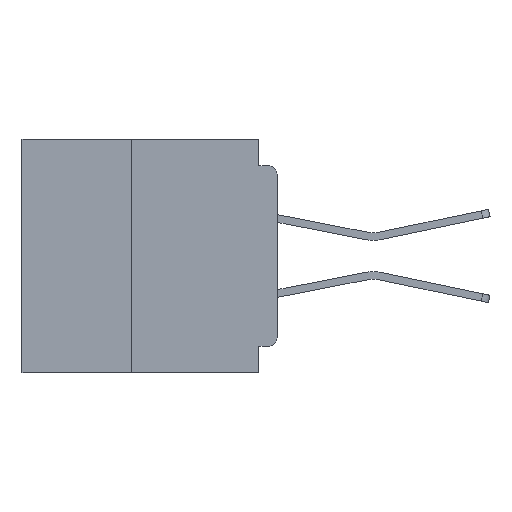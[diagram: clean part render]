
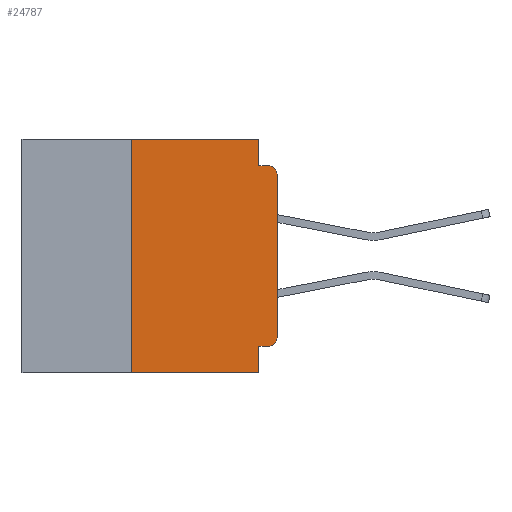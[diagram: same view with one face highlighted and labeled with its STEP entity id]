
A CAD part, left-side view. The second image highlights one B-rep face of the part: STEP entity #24787.
In plain terms, the highlighted planar face has unit normal (-1, 0, 0).
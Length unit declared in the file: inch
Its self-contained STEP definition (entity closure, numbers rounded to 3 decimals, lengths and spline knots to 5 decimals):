
#1979 = VECTOR ( 'NONE', #18012, 39.37008 ) ;
#2396 = EDGE_CURVE ( 'NONE', #15850, #34930, #3824, .T. ) ;
#2592 = VERTEX_POINT ( 'NONE', #10061 ) ;
#2812 = VECTOR ( 'NONE', #30280, 39.37008 ) ;
#2983 = DIRECTION ( 'NONE',  ( 0., -1., 0. ) ) ;
#3063 = ORIENTED_EDGE ( 'NONE', *, *, #26217, .F. ) ;
#3742 = DIRECTION ( 'NONE',  ( 0., -1., 0. ) ) ;
#3824 = LINE ( 'NONE', #6038, #18652 ) ;
#4009 = ORIENTED_EDGE ( 'NONE', *, *, #22475, .F. ) ;
#4136 = DIRECTION ( 'NONE',  ( 0., 0., 1. ) ) ;
#5401 = EDGE_CURVE ( 'NONE', #19291, #34097, #37552, .T. ) ;
#5407 = LINE ( 'NONE', #26726, #20202 ) ;
#5460 = VECTOR ( 'NONE', #17049, 39.37008 ) ;
#5598 = FACE_OUTER_BOUND ( 'NONE', #36679, .T. ) ;
#5671 = CIRCLE ( 'NONE', #7348, 0.015 ) ;
#5683 = VERTEX_POINT ( 'NONE', #23159 ) ;
#5840 = EDGE_CURVE ( 'NONE', #33795, #24374, #13364, .T. ) ;
#5862 = ORIENTED_EDGE ( 'NONE', *, *, #24392, .F. ) ;
#6038 = CARTESIAN_POINT ( 'NONE',  ( 0., 0., -0.045 ) ) ;
#6291 = AXIS2_PLACEMENT_3D ( 'NONE', #11101, #31573, #14049 ) ;
#7348 = AXIS2_PLACEMENT_3D ( 'NONE', #16916, #37301, #19865 ) ;
#8379 = EDGE_CURVE ( 'NONE', #2592, #34930, #5671, .T. ) ;
#8705 = ORIENTED_EDGE ( 'NONE', *, *, #24047, .T. ) ;
#8788 = VECTOR ( 'NONE', #3742, 39.37008 ) ;
#8977 = CIRCLE ( 'NONE', #6291, 0.015 ) ;
#10061 = CARTESIAN_POINT ( 'NONE',  ( 0., 0., -0.06 ) ) ;
#11101 = CARTESIAN_POINT ( 'NONE',  ( 0., 0.015, -0.34 ) ) ;
#11539 = DIRECTION ( 'NONE',  ( 0., 0., -1. ) ) ;
#13364 = LINE ( 'NONE', #17894, #5460 ) ;
#13857 = EDGE_CURVE ( 'NONE', #27856, #2592, #37462, .T. ) ;
#14049 = DIRECTION ( 'NONE',  ( 0., 0., -1. ) ) ;
#15850 = VERTEX_POINT ( 'NONE', #20025 ) ;
#16067 = ORIENTED_EDGE ( 'NONE', *, *, #28334, .F. ) ;
#16609 = LINE ( 'NONE', #24405, #8788 ) ;
#16916 = CARTESIAN_POINT ( 'NONE',  ( 0., 0.015, -0.06 ) ) ;
#17049 = DIRECTION ( 'NONE',  ( 0., 1., 0. ) ) ;
#17316 = CARTESIAN_POINT ( 'NONE',  ( 0., 0.437, 0. ) ) ;
#17766 = LINE ( 'NONE', #23648, #1979 ) ;
#17894 = CARTESIAN_POINT ( 'NONE',  ( 0., 0., -0.355 ) ) ;
#18012 = DIRECTION ( 'NONE',  ( 0., 0., 1. ) ) ;
#18411 = CARTESIAN_POINT ( 'NONE',  ( 0., 0.031, -0.355 ) ) ;
#18652 = VECTOR ( 'NONE', #2983, 39.37008 ) ;
#19257 = ORIENTED_EDGE ( 'NONE', *, *, #13857, .T. ) ;
#19291 = VERTEX_POINT ( 'NONE', #37078 ) ;
#19865 = DIRECTION ( 'NONE',  ( 0., 0., -1. ) ) ;
#20025 = CARTESIAN_POINT ( 'NONE',  ( 0., 0.031, -0.045 ) ) ;
#20202 = VECTOR ( 'NONE', #23793, 39.37008 ) ;
#20294 = PLANE ( 'NONE',  #26511 ) ;
#21119 = ORIENTED_EDGE ( 'NONE', *, *, #2396, .F. ) ;
#21906 = CARTESIAN_POINT ( 'NONE',  ( 0., 0.031, -0.4 ) ) ;
#22475 = EDGE_CURVE ( 'NONE', #19291, #5683, #17766, .T. ) ;
#23159 = CARTESIAN_POINT ( 'NONE',  ( 0., 0.25, 0. ) ) ;
#23648 = CARTESIAN_POINT ( 'NONE',  ( 0., 0.25, -0.4 ) ) ;
#23793 = DIRECTION ( 'NONE',  ( 0., 0., -1. ) ) ;
#24047 = EDGE_CURVE ( 'NONE', #33795, #27856, #8977, .T. ) ;
#24374 = VERTEX_POINT ( 'NONE', #18411 ) ;
#24392 = EDGE_CURVE ( 'NONE', #24374, #34097, #26375, .T. ) ;
#24405 = CARTESIAN_POINT ( 'NONE',  ( 0., 0.437, 0. ) ) ;
#24787 = ADVANCED_FACE ( 'NONE', ( #5598 ), #20294, .F. ) ;
#24788 = VERTEX_POINT ( 'NONE', #26175 ) ;
#26175 = CARTESIAN_POINT ( 'NONE',  ( 0., 0.031, 0. ) ) ;
#26217 = EDGE_CURVE ( 'NONE', #5683, #24788, #16609, .T. ) ;
#26375 = LINE ( 'NONE', #27344, #2812 ) ;
#26381 = CARTESIAN_POINT ( 'NONE',  ( 0., 0.015, -0.355 ) ) ;
#26511 = AXIS2_PLACEMENT_3D ( 'NONE', #17316, #29076, #11539 ) ;
#26726 = CARTESIAN_POINT ( 'NONE',  ( 0., 0.031, 0. ) ) ;
#27344 = CARTESIAN_POINT ( 'NONE',  ( 0., 0.031, -0.4 ) ) ;
#27856 = VERTEX_POINT ( 'NONE', #30460 ) ;
#28334 = EDGE_CURVE ( 'NONE', #24788, #15850, #5407, .T. ) ;
#29076 = DIRECTION ( 'NONE',  ( 1., 0., 0. ) ) ;
#29760 = VECTOR ( 'NONE', #4136, 39.37008 ) ;
#29866 = VECTOR ( 'NONE', #33518, 39.37008 ) ;
#30280 = DIRECTION ( 'NONE',  ( 0., 0., -1. ) ) ;
#30460 = CARTESIAN_POINT ( 'NONE',  ( 0., 0., -0.34 ) ) ;
#31173 = ORIENTED_EDGE ( 'NONE', *, *, #5840, .F. ) ;
#31573 = DIRECTION ( 'NONE',  ( -1., 0., 0. ) ) ;
#33518 = DIRECTION ( 'NONE',  ( 0., -1., 0. ) ) ;
#33681 = CARTESIAN_POINT ( 'NONE',  ( 0., 0.437, -0.4 ) ) ;
#33686 = CARTESIAN_POINT ( 'NONE',  ( 0., 0., 0. ) ) ;
#33795 = VERTEX_POINT ( 'NONE', #26381 ) ;
#34097 = VERTEX_POINT ( 'NONE', #21906 ) ;
#34930 = VERTEX_POINT ( 'NONE', #37336 ) ;
#35732 = ORIENTED_EDGE ( 'NONE', *, *, #8379, .T. ) ;
#36197 = ORIENTED_EDGE ( 'NONE', *, *, #5401, .T. ) ;
#36679 = EDGE_LOOP ( 'NONE', ( #19257, #35732, #21119, #16067, #3063, #4009, #36197, #5862, #31173, #8705 ) ) ;
#37078 = CARTESIAN_POINT ( 'NONE',  ( 0., 0.25, -0.4 ) ) ;
#37301 = DIRECTION ( 'NONE',  ( -1., 0., 0. ) ) ;
#37336 = CARTESIAN_POINT ( 'NONE',  ( 0., 0.015, -0.045 ) ) ;
#37462 = LINE ( 'NONE', #33686, #29760 ) ;
#37552 = LINE ( 'NONE', #33681, #29866 ) ;
